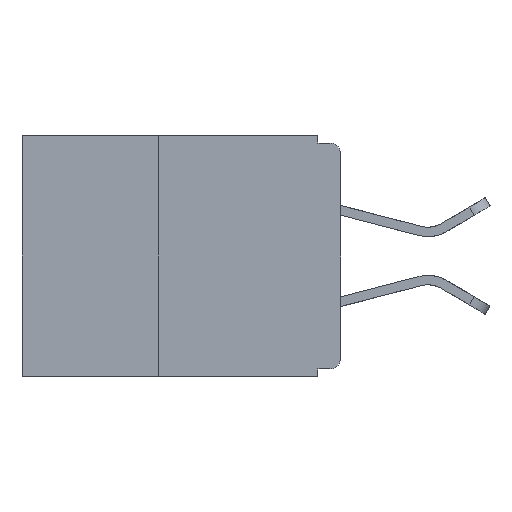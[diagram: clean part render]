
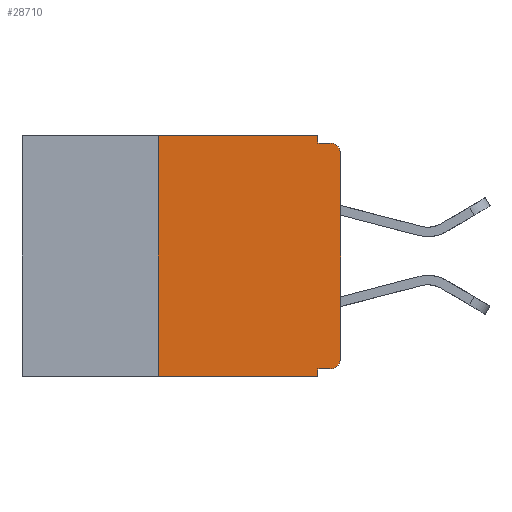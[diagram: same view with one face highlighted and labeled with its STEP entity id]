
A CAD part, left-side view. The second image highlights one B-rep face of the part: STEP entity #28710.
In plain terms, the highlighted planar face has unit normal (-1, 0, 0).
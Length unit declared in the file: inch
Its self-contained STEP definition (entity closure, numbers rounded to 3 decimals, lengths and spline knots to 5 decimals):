
#344 = VECTOR ( 'NONE', #3063, 39.37008 ) ;
#534 = VERTEX_POINT ( 'NONE', #28331 ) ;
#790 = VECTOR ( 'NONE', #10628, 39.37008 ) ;
#853 = CARTESIAN_POINT ( 'NONE',  ( 0., 0.031, -0.33 ) ) ;
#921 = CARTESIAN_POINT ( 'NONE',  ( 0., 0.437, -0.33 ) ) ;
#2499 = DIRECTION ( 'NONE',  ( 0., 0., 1. ) ) ;
#2866 = DIRECTION ( 'NONE',  ( 0., 0., -1. ) ) ;
#3063 = DIRECTION ( 'NONE',  ( 0., 0., -1. ) ) ;
#3123 = EDGE_CURVE ( 'NONE', #7905, #23335, #24960, .T. ) ;
#3387 = EDGE_CURVE ( 'NONE', #13085, #23577, #5545, .T. ) ;
#3429 = CARTESIAN_POINT ( 'NONE',  ( 0., 0., -0.32 ) ) ;
#4417 = CARTESIAN_POINT ( 'NONE',  ( 0., 0., -0.025 ) ) ;
#4612 = LINE ( 'NONE', #16973, #23691 ) ;
#5228 = PLANE ( 'NONE',  #30633 ) ;
#5323 = CIRCLE ( 'NONE', #12026, 0.015 ) ;
#5545 = CIRCLE ( 'NONE', #9111, 0.015 ) ;
#6515 = LINE ( 'NONE', #27155, #790 ) ;
#6926 = EDGE_CURVE ( 'NONE', #23577, #17130, #6515, .T. ) ;
#6953 = ORIENTED_EDGE ( 'NONE', *, *, #25260, .F. ) ;
#7511 = EDGE_LOOP ( 'NONE', ( #17006, #19917, #26261, #28474, #19627, #6953, #26819, #10519, #24563, #14348 ) ) ;
#7905 = VERTEX_POINT ( 'NONE', #19224 ) ;
#8115 = EDGE_CURVE ( 'NONE', #23335, #534, #30622, .T. ) ;
#8184 = VERTEX_POINT ( 'NONE', #853 ) ;
#8516 = CARTESIAN_POINT ( 'NONE',  ( 0., 0., -0.01 ) ) ;
#9111 = AXIS2_PLACEMENT_3D ( 'NONE', #28115, #28078, #27986 ) ;
#9484 = CARTESIAN_POINT ( 'NONE',  ( 0., 0., -0.305 ) ) ;
#9965 = DIRECTION ( 'NONE',  ( 0., -1., 0. ) ) ;
#10002 = CARTESIAN_POINT ( 'NONE',  ( 0., 0.437, 0. ) ) ;
#10378 = CARTESIAN_POINT ( 'NONE',  ( 0., 0.015, -0.01 ) ) ;
#10519 = ORIENTED_EDGE ( 'NONE', *, *, #25961, .F. ) ;
#10628 = DIRECTION ( 'NONE',  ( 0., 0., 1. ) ) ;
#10751 = DIRECTION ( 'NONE',  ( -1., 0., 0. ) ) ;
#11164 = EDGE_CURVE ( 'NONE', #534, #20685, #27479, .T. ) ;
#12026 = AXIS2_PLACEMENT_3D ( 'NONE', #24918, #10751, #27276 ) ;
#13085 = VERTEX_POINT ( 'NONE', #29787 ) ;
#13646 = EDGE_CURVE ( 'NONE', #24899, #8184, #30292, .T. ) ;
#14348 = ORIENTED_EDGE ( 'NONE', *, *, #3387, .T. ) ;
#15006 = EDGE_CURVE ( 'NONE', #13085, #18281, #23907, .T. ) ;
#15115 = CARTESIAN_POINT ( 'NONE',  ( 0., 0.031, 0. ) ) ;
#15535 = CARTESIAN_POINT ( 'NONE',  ( 0., 0.25, -0.33 ) ) ;
#16973 = CARTESIAN_POINT ( 'NONE',  ( 0., 0.25, -0.33 ) ) ;
#17006 = ORIENTED_EDGE ( 'NONE', *, *, #6926, .T. ) ;
#17130 = VERTEX_POINT ( 'NONE', #4417 ) ;
#17150 = CARTESIAN_POINT ( 'NONE',  ( 0., 0.031, -0.33 ) ) ;
#17358 = DIRECTION ( 'NONE',  ( 1., 0., 0. ) ) ;
#18281 = VERTEX_POINT ( 'NONE', #25829 ) ;
#18766 = VECTOR ( 'NONE', #9965, 39.37008 ) ;
#19224 = CARTESIAN_POINT ( 'NONE',  ( 0., 0.25, 0. ) ) ;
#19627 = ORIENTED_EDGE ( 'NONE', *, *, #3123, .F. ) ;
#19917 = ORIENTED_EDGE ( 'NONE', *, *, #21444, .T. ) ;
#20206 = DIRECTION ( 'NONE',  ( 0., -1., 0. ) ) ;
#20535 = VECTOR ( 'NONE', #25008, 39.37008 ) ;
#20685 = VERTEX_POINT ( 'NONE', #10378 ) ;
#20933 = FACE_OUTER_BOUND ( 'NONE', #7511, .T. ) ;
#21444 = EDGE_CURVE ( 'NONE', #17130, #20685, #5323, .T. ) ;
#21693 = DIRECTION ( 'NONE',  ( 0., 0., -1. ) ) ;
#21979 = CARTESIAN_POINT ( 'NONE',  ( 0., 0.437, 0. ) ) ;
#22650 = DIRECTION ( 'NONE',  ( 0., 1., 0. ) ) ;
#23282 = VECTOR ( 'NONE', #20206, 39.37008 ) ;
#23335 = VERTEX_POINT ( 'NONE', #27396 ) ;
#23577 = VERTEX_POINT ( 'NONE', #9484 ) ;
#23691 = VECTOR ( 'NONE', #2499, 39.37008 ) ;
#23907 = LINE ( 'NONE', #3429, #28698 ) ;
#23996 = LINE ( 'NONE', #17150, #25495 ) ;
#24563 = ORIENTED_EDGE ( 'NONE', *, *, #15006, .F. ) ;
#24899 = VERTEX_POINT ( 'NONE', #15535 ) ;
#24918 = CARTESIAN_POINT ( 'NONE',  ( 0., 0.015, -0.025 ) ) ;
#24960 = LINE ( 'NONE', #10002, #18766 ) ;
#25008 = DIRECTION ( 'NONE',  ( 0., -1., 0. ) ) ;
#25260 = EDGE_CURVE ( 'NONE', #24899, #7905, #4612, .T. ) ;
#25495 = VECTOR ( 'NONE', #21693, 39.37008 ) ;
#25829 = CARTESIAN_POINT ( 'NONE',  ( 0., 0.031, -0.32 ) ) ;
#25961 = EDGE_CURVE ( 'NONE', #18281, #8184, #23996, .T. ) ;
#26261 = ORIENTED_EDGE ( 'NONE', *, *, #11164, .F. ) ;
#26819 = ORIENTED_EDGE ( 'NONE', *, *, #13646, .T. ) ;
#27155 = CARTESIAN_POINT ( 'NONE',  ( 0., 0., 0. ) ) ;
#27276 = DIRECTION ( 'NONE',  ( 0., 0., -1. ) ) ;
#27396 = CARTESIAN_POINT ( 'NONE',  ( 0., 0.031, 0. ) ) ;
#27479 = LINE ( 'NONE', #8516, #20535 ) ;
#27986 = DIRECTION ( 'NONE',  ( 0., 0., -1. ) ) ;
#28078 = DIRECTION ( 'NONE',  ( -1., 0., 0. ) ) ;
#28115 = CARTESIAN_POINT ( 'NONE',  ( 0., 0.015, -0.305 ) ) ;
#28331 = CARTESIAN_POINT ( 'NONE',  ( 0., 0.031, -0.01 ) ) ;
#28474 = ORIENTED_EDGE ( 'NONE', *, *, #8115, .F. ) ;
#28698 = VECTOR ( 'NONE', #22650, 39.37008 ) ;
#28710 = ADVANCED_FACE ( 'NONE', ( #20933 ), #5228, .F. ) ;
#29787 = CARTESIAN_POINT ( 'NONE',  ( 0., 0.015, -0.32 ) ) ;
#30292 = LINE ( 'NONE', #921, #23282 ) ;
#30622 = LINE ( 'NONE', #15115, #344 ) ;
#30633 = AXIS2_PLACEMENT_3D ( 'NONE', #21979, #17358, #2866 ) ;
